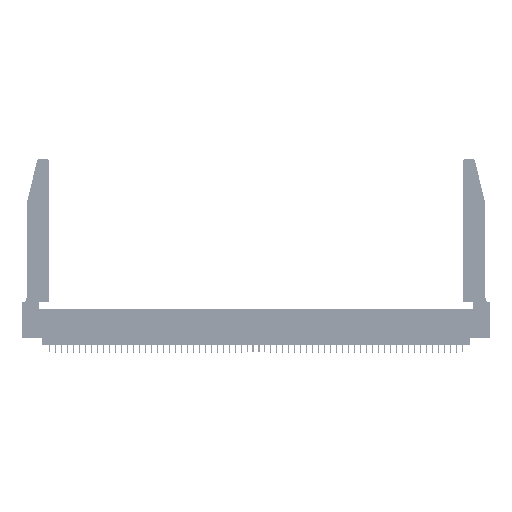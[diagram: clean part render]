
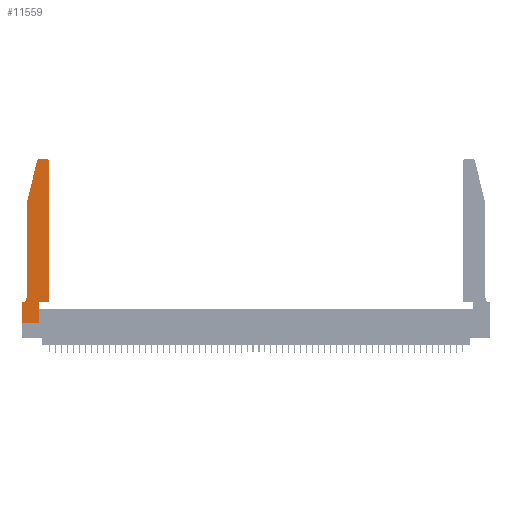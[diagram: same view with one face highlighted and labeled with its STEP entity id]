
A CAD part, top view. The second image highlights one B-rep face of the part: STEP entity #11559.
In plain terms, the highlighted planar face has unit normal (0, 0, 1).
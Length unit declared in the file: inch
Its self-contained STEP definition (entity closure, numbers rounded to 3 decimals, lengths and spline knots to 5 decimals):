
#254 = LINE ( 'NONE', #34973, #51761 ) ;
#2011 = CARTESIAN_POINT ( 'NONE',  ( 0., 0., 0.37 ) ) ;
#2195 = DIRECTION ( 'NONE',  ( 1., 0., 0. ) ) ;
#2301 = VECTOR ( 'NONE', #19798, 39.37008 ) ;
#2326 = ORIENTED_EDGE ( 'NONE', *, *, #35686, .T. ) ;
#3509 = EDGE_CURVE ( 'NONE', #38298, #15989, #16816, .T. ) ;
#4005 = CARTESIAN_POINT ( 'NONE',  ( 0.2605, 2.75, 0.37 ) ) ;
#4174 = EDGE_LOOP ( 'NONE', ( #50652, #11093, #14184, #34794, #17340, #40661, #31672, #2326, #5068, #23961, #9249, #19909 ) ) ;
#4534 = VERTEX_POINT ( 'NONE', #26812 ) ;
#5068 = ORIENTED_EDGE ( 'NONE', *, *, #26497, .T. ) ;
#6222 = CARTESIAN_POINT ( 'NONE',  ( 0.4205, 2.72, 0.37 ) ) ;
#7039 = DIRECTION ( 'NONE',  ( 1., 0., 0. ) ) ;
#7575 = CARTESIAN_POINT ( 'NONE',  ( 0.2865, 0., 0.37 ) ) ;
#8854 = CARTESIAN_POINT ( 'NONE',  ( 0.0755, 0.35, 0.37 ) ) ;
#8919 = CARTESIAN_POINT ( 'NONE',  ( 0.0755, 0.42, 0.37 ) ) ;
#9249 = ORIENTED_EDGE ( 'NONE', *, *, #41993, .T. ) ;
#9959 = DIRECTION ( 'NONE',  ( 1., 0., 0. ) ) ;
#10024 = VERTEX_POINT ( 'NONE', #16248 ) ;
#10171 = VECTOR ( 'NONE', #12543, 39.37008 ) ;
#10923 = AXIS2_PLACEMENT_3D ( 'NONE', #45933, #41411, #7039 ) ;
#11093 = ORIENTED_EDGE ( 'NONE', *, *, #16823, .T. ) ;
#11182 = VERTEX_POINT ( 'NONE', #32169 ) ;
#11559 = ADVANCED_FACE ( 'NONE', ( #44318 ), #15337, .T. ) ;
#11826 = EDGE_CURVE ( 'NONE', #4534, #14200, #12471, .T. ) ;
#11897 = DIRECTION ( 'NONE',  ( 0., 0., -1. ) ) ;
#12238 = LINE ( 'NONE', #34412, #36879 ) ;
#12471 = LINE ( 'NONE', #17304, #46868 ) ;
#12543 = DIRECTION ( 'NONE',  ( -1., 0., 0. ) ) ;
#13719 = EDGE_CURVE ( 'NONE', #15989, #49082, #32585, .T. ) ;
#14184 = ORIENTED_EDGE ( 'NONE', *, *, #24560, .T. ) ;
#14200 = VERTEX_POINT ( 'NONE', #8919 ) ;
#14769 = DIRECTION ( 'NONE',  ( 0., 0., 1. ) ) ;
#15337 = PLANE ( 'NONE',  #54126 ) ;
#15806 = EDGE_CURVE ( 'NONE', #11182, #18912, #29586, .T. ) ;
#15989 = VERTEX_POINT ( 'NONE', #36916 ) ;
#16248 = CARTESIAN_POINT ( 'NONE',  ( 0.4505, 2.72, 0.37 ) ) ;
#16816 = LINE ( 'NONE', #8854, #10171 ) ;
#16823 = EDGE_CURVE ( 'NONE', #18912, #27626, #25421, .T. ) ;
#17304 = CARTESIAN_POINT ( 'NONE',  ( 0.0755, 2., 0.37 ) ) ;
#17340 = ORIENTED_EDGE ( 'NONE', *, *, #38417, .T. ) ;
#18912 = VERTEX_POINT ( 'NONE', #48399 ) ;
#19282 = DIRECTION ( 'NONE',  ( 0., 0., 1. ) ) ;
#19798 = DIRECTION ( 'NONE',  ( 0., -1., 0. ) ) ;
#19909 = ORIENTED_EDGE ( 'NONE', *, *, #34581, .T. ) ;
#20470 = CARTESIAN_POINT ( 'NONE',  ( 0.2865, 0.35, 0.37 ) ) ;
#21496 = VERTEX_POINT ( 'NONE', #20470 ) ;
#22743 = CARTESIAN_POINT ( 'NONE',  ( 0., 0.35, 0.37 ) ) ;
#23961 = ORIENTED_EDGE ( 'NONE', *, *, #39515, .T. ) ;
#24079 = DIRECTION ( 'NONE',  ( -0.239, -0.971, 0. ) ) ;
#24438 = VECTOR ( 'NONE', #34701, 39.37008 ) ;
#24560 = EDGE_CURVE ( 'NONE', #27626, #4534, #33195, .T. ) ;
#25250 = DIRECTION ( 'NONE',  ( -1., 0., 0. ) ) ;
#25421 = CIRCLE ( 'NONE', #10923, 0.03 ) ;
#25965 = DIRECTION ( 'NONE',  ( 1., 0., 0. ) ) ;
#26497 = EDGE_CURVE ( 'NONE', #38901, #21496, #54292, .T. ) ;
#26812 = CARTESIAN_POINT ( 'NONE',  ( 0.0755, 2., 0.37 ) ) ;
#27626 = VERTEX_POINT ( 'NONE', #47586 ) ;
#27679 = VECTOR ( 'NONE', #24079, 39.37008 ) ;
#29567 = DIRECTION ( 'NONE',  ( 1., 0., 0. ) ) ;
#29586 = LINE ( 'NONE', #4005, #24438 ) ;
#30098 = VERTEX_POINT ( 'NONE', #37755 ) ;
#30218 = CARTESIAN_POINT ( 'NONE',  ( 0.4505, 0.35, 0.37 ) ) ;
#31672 = ORIENTED_EDGE ( 'NONE', *, *, #13719, .T. ) ;
#32169 = CARTESIAN_POINT ( 'NONE',  ( 0.4205, 2.75, 0.37 ) ) ;
#32562 = VECTOR ( 'NONE', #25965, 39.37008 ) ;
#32585 = LINE ( 'NONE', #32858, #2301 ) ;
#32858 = CARTESIAN_POINT ( 'NONE',  ( 0., 0., 0.37 ) ) ;
#33195 = LINE ( 'NONE', #42250, #27679 ) ;
#33956 = LINE ( 'NONE', #30218, #32562 ) ;
#34412 = CARTESIAN_POINT ( 'NONE',  ( 0., 0., 0.37 ) ) ;
#34581 = EDGE_CURVE ( 'NONE', #10024, #11182, #47661, .T. ) ;
#34701 = DIRECTION ( 'NONE',  ( -1., 0., 0. ) ) ;
#34794 = ORIENTED_EDGE ( 'NONE', *, *, #11826, .T. ) ;
#34973 = CARTESIAN_POINT ( 'NONE',  ( 0.4505, 0.35, 0.37 ) ) ;
#35212 = CIRCLE ( 'NONE', #37896, 0.07 ) ;
#35686 = EDGE_CURVE ( 'NONE', #49082, #38901, #12238, .T. ) ;
#36689 = CARTESIAN_POINT ( 'NONE',  ( 0.2865, 0.35, 0.37 ) ) ;
#36879 = VECTOR ( 'NONE', #29567, 39.37008 ) ;
#36916 = CARTESIAN_POINT ( 'NONE',  ( 0., 0.35, 0.37 ) ) ;
#37684 = VECTOR ( 'NONE', #54010, 39.37008 ) ;
#37755 = CARTESIAN_POINT ( 'NONE',  ( 0.4505, 0.35, 0.37 ) ) ;
#37896 = AXIS2_PLACEMENT_3D ( 'NONE', #48872, #11897, #25250 ) ;
#38298 = VERTEX_POINT ( 'NONE', #40327 ) ;
#38417 = EDGE_CURVE ( 'NONE', #14200, #38298, #35212, .T. ) ;
#38901 = VERTEX_POINT ( 'NONE', #7575 ) ;
#39515 = EDGE_CURVE ( 'NONE', #21496, #30098, #33956, .T. ) ;
#40327 = CARTESIAN_POINT ( 'NONE',  ( 0.0055, 0.35, 0.37 ) ) ;
#40661 = ORIENTED_EDGE ( 'NONE', *, *, #3509, .T. ) ;
#41411 = DIRECTION ( 'NONE',  ( 0., 0., 1. ) ) ;
#41993 = EDGE_CURVE ( 'NONE', #30098, #10024, #254, .T. ) ;
#42250 = CARTESIAN_POINT ( 'NONE',  ( 0.0755, 2., 0.37 ) ) ;
#43109 = DIRECTION ( 'NONE',  ( 0., -1., 0. ) ) ;
#44318 = FACE_OUTER_BOUND ( 'NONE', #4174, .T. ) ;
#45933 = CARTESIAN_POINT ( 'NONE',  ( 0.284, 2.72, 0.37 ) ) ;
#46868 = VECTOR ( 'NONE', #43109, 39.37008 ) ;
#47586 = CARTESIAN_POINT ( 'NONE',  ( 0.25487, 2.72718, 0.37 ) ) ;
#47661 = CIRCLE ( 'NONE', #49508, 0.03 ) ;
#48399 = CARTESIAN_POINT ( 'NONE',  ( 0.284, 2.75, 0.37 ) ) ;
#48872 = CARTESIAN_POINT ( 'NONE',  ( 0.0055, 0.42, 0.37 ) ) ;
#49082 = VERTEX_POINT ( 'NONE', #2011 ) ;
#49508 = AXIS2_PLACEMENT_3D ( 'NONE', #6222, #19282, #2195 ) ;
#50652 = ORIENTED_EDGE ( 'NONE', *, *, #15806, .T. ) ;
#51761 = VECTOR ( 'NONE', #52274, 39.37008 ) ;
#52274 = DIRECTION ( 'NONE',  ( 0., 1., 0. ) ) ;
#54010 = DIRECTION ( 'NONE',  ( 0., 1., 0. ) ) ;
#54126 = AXIS2_PLACEMENT_3D ( 'NONE', #22743, #14769, #9959 ) ;
#54292 = LINE ( 'NONE', #36689, #37684 ) ;
